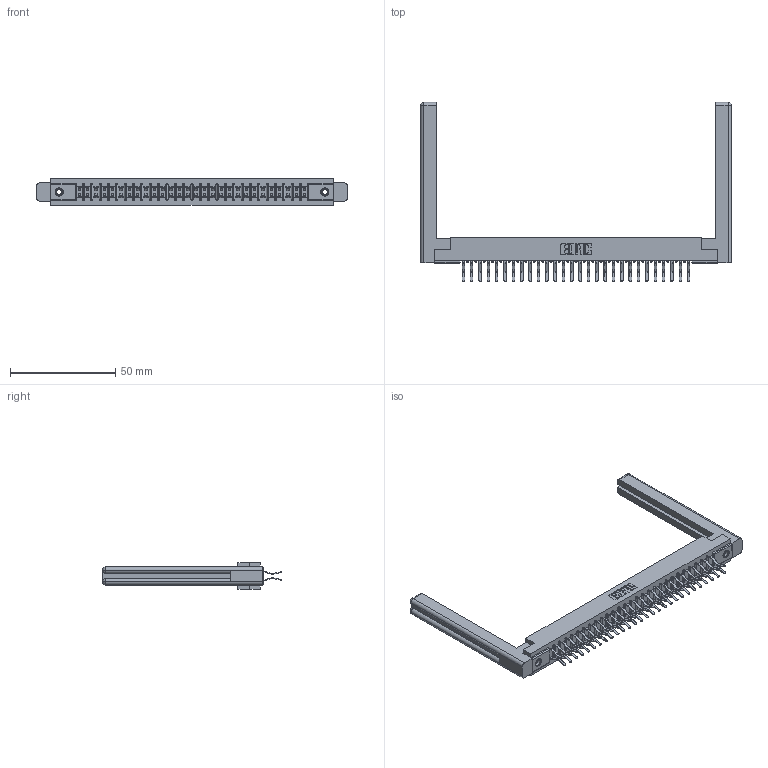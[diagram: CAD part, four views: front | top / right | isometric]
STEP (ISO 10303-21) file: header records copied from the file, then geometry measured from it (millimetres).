
FILE_DESCRIPTION (( 'STEP AP203' ), '1' );
FILE_NAME ('357-056-560-258.STEP', '2019-09-19T05:05:09', ( '' ), ( '' ), 'SwSTEP 2.0', 'SolidWorks 2016', '' );
FILE_SCHEMA (( 'CONFIG_CONTROL_DESIGN' ));
Length unit declared in the file: inch
Products named in the file (5): 357-056-560-258; 345-250-001_345-250-001-102; 307-220-058; 307-290-001_560; 307 Part_.156 Dia Mounting Holes
Assembly tree (61 placements, depth 2):
  357-056-560-258
    307 Part_.156 Dia Mounting Holes
    307-290-001_560  x56
    307-220-058  x2
    345-250-001_345-250-001-102  x2
Bounding box: 147.57 x 85.04 x 12.7 mm (x, y, z)
Volume: 22792.7 mm3; surface area: 24151.7 mm2
Topology: 61 solids, 61 shells, 3089 faces, 8629 edges, 5586 vertices
Faces by surface type: plane 2002, cylinder 1005, sphere 58, torus 12, cone 12
Entity records: 29363 total; most frequent: CARTESIAN_POINT 4827, ORIENTED_EDGE 4724, DIRECTION 4692, EDGE_CURVE 2362, LINE 1802, VECTOR 1802, VERTEX_POINT 1526, AXIS2_PLACEMENT_3D 1445
